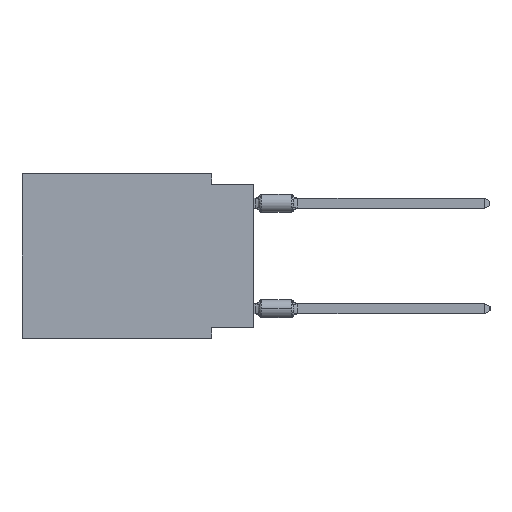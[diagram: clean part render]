
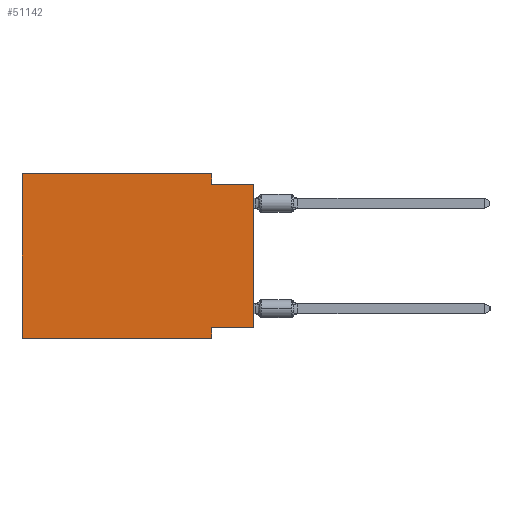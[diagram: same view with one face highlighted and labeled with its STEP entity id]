
A CAD part, left-side view. The second image highlights one B-rep face of the part: STEP entity #51142.
In plain terms, the highlighted planar face has unit normal (-1, 0, 0).
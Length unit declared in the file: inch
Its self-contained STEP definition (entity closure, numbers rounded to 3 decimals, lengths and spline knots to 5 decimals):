
#479 = VERTEX_POINT ( 'NONE', #42170 ) ;
#579 = CARTESIAN_POINT ( 'NONE',  ( 0., 0.1, 0. ) ) ;
#1050 = VERTEX_POINT ( 'NONE', #13389 ) ;
#4657 = CARTESIAN_POINT ( 'NONE',  ( 0., 0.55, -0.39 ) ) ;
#6188 = DIRECTION ( 'NONE',  ( 0., 0., 1. ) ) ;
#7927 = LINE ( 'NONE', #51828, #45208 ) ;
#8073 = ORIENTED_EDGE ( 'NONE', *, *, #20036, .F. ) ;
#10201 = LINE ( 'NONE', #579, #53583 ) ;
#10935 = CARTESIAN_POINT ( 'NONE',  ( 0., 0.1, -0.39 ) ) ;
#10939 = ORIENTED_EDGE ( 'NONE', *, *, #23454, .F. ) ;
#11357 = DIRECTION ( 'NONE',  ( 0., 0., -1. ) ) ;
#12221 = AXIS2_PLACEMENT_3D ( 'NONE', #15758, #51443, #11357 ) ;
#12731 = CARTESIAN_POINT ( 'NONE',  ( 0., 0.1, -0.365 ) ) ;
#13389 = CARTESIAN_POINT ( 'NONE',  ( 0., 0.1, -0.025 ) ) ;
#13759 = VECTOR ( 'NONE', #46853, 39.37008 ) ;
#15005 = CARTESIAN_POINT ( 'NONE',  ( 0., 0.1, -0.39 ) ) ;
#15758 = CARTESIAN_POINT ( 'NONE',  ( 0., 0.55, 0. ) ) ;
#16123 = DIRECTION ( 'NONE',  ( 0., 0., 1. ) ) ;
#17072 = VERTEX_POINT ( 'NONE', #50886 ) ;
#17306 = EDGE_LOOP ( 'NONE', ( #43829, #41754, #8073, #39857, #32442, #53621, #10939, #44395 ) ) ;
#18512 = VERTEX_POINT ( 'NONE', #30689 ) ;
#20036 = EDGE_CURVE ( 'NONE', #18512, #1050, #10201, .T. ) ;
#20108 = CARTESIAN_POINT ( 'NONE',  ( 0., 0., -0.025 ) ) ;
#22002 = VECTOR ( 'NONE', #6188, 39.37008 ) ;
#23454 = EDGE_CURVE ( 'NONE', #43444, #30360, #50428, .T. ) ;
#23793 = LINE ( 'NONE', #27915, #28228 ) ;
#26973 = CARTESIAN_POINT ( 'NONE',  ( 0., 0.55, -0.39 ) ) ;
#27870 = CARTESIAN_POINT ( 'NONE',  ( 0., 0.55, 0. ) ) ;
#27915 = CARTESIAN_POINT ( 'NONE',  ( 0., 0., -0.365 ) ) ;
#28228 = VECTOR ( 'NONE', #54254, 39.37008 ) ;
#29016 = LINE ( 'NONE', #33385, #50928 ) ;
#30360 = VERTEX_POINT ( 'NONE', #10935 ) ;
#30689 = CARTESIAN_POINT ( 'NONE',  ( 0., 0.1, 0. ) ) ;
#32442 = ORIENTED_EDGE ( 'NONE', *, *, #44029, .F. ) ;
#32848 = DIRECTION ( 'NONE',  ( 0., 0., -1. ) ) ;
#32992 = DIRECTION ( 'NONE',  ( 0., 0., -1. ) ) ;
#33385 = CARTESIAN_POINT ( 'NONE',  ( 0., 0., 0. ) ) ;
#33957 = CARTESIAN_POINT ( 'NONE',  ( 0., 0., -0.025 ) ) ;
#34355 = EDGE_CURVE ( 'NONE', #38635, #30360, #48612, .T. ) ;
#38004 = FACE_OUTER_BOUND ( 'NONE', #17306, .T. ) ;
#38635 = VERTEX_POINT ( 'NONE', #4657 ) ;
#38823 = VERTEX_POINT ( 'NONE', #20108 ) ;
#39857 = ORIENTED_EDGE ( 'NONE', *, *, #53660, .F. ) ;
#40358 = EDGE_CURVE ( 'NONE', #479, #43444, #23793, .T. ) ;
#41754 = ORIENTED_EDGE ( 'NONE', *, *, #48112, .F. ) ;
#42170 = CARTESIAN_POINT ( 'NONE',  ( 0., 0., -0.365 ) ) ;
#42923 = VECTOR ( 'NONE', #49208, 39.37008 ) ;
#43444 = VERTEX_POINT ( 'NONE', #12731 ) ;
#43829 = ORIENTED_EDGE ( 'NONE', *, *, #44090, .T. ) ;
#44029 = EDGE_CURVE ( 'NONE', #38635, #17072, #46286, .T. ) ;
#44090 = EDGE_CURVE ( 'NONE', #479, #38823, #29016, .T. ) ;
#44395 = ORIENTED_EDGE ( 'NONE', *, *, #40358, .F. ) ;
#45208 = VECTOR ( 'NONE', #47737, 39.37008 ) ;
#46286 = LINE ( 'NONE', #27870, #22002 ) ;
#46853 = DIRECTION ( 'NONE',  ( 0., -1., 0. ) ) ;
#47737 = DIRECTION ( 'NONE',  ( 0., -1., 0. ) ) ;
#48112 = EDGE_CURVE ( 'NONE', #1050, #38823, #55920, .T. ) ;
#48612 = LINE ( 'NONE', #26973, #42923 ) ;
#49208 = DIRECTION ( 'NONE',  ( 0., -1., 0. ) ) ;
#50428 = LINE ( 'NONE', #15005, #51547 ) ;
#50886 = CARTESIAN_POINT ( 'NONE',  ( 0., 0.55, 0. ) ) ;
#50928 = VECTOR ( 'NONE', #16123, 39.37008 ) ;
#51142 = ADVANCED_FACE ( 'NONE', ( #38004 ), #55843, .F. ) ;
#51443 = DIRECTION ( 'NONE',  ( 1., 0., 0. ) ) ;
#51547 = VECTOR ( 'NONE', #32848, 39.37008 ) ;
#51828 = CARTESIAN_POINT ( 'NONE',  ( 0., 0.55, 0. ) ) ;
#53583 = VECTOR ( 'NONE', #32992, 39.37008 ) ;
#53621 = ORIENTED_EDGE ( 'NONE', *, *, #34355, .T. ) ;
#53660 = EDGE_CURVE ( 'NONE', #17072, #18512, #7927, .T. ) ;
#54254 = DIRECTION ( 'NONE',  ( 0., 1., 0. ) ) ;
#55843 = PLANE ( 'NONE',  #12221 ) ;
#55920 = LINE ( 'NONE', #33957, #13759 ) ;
